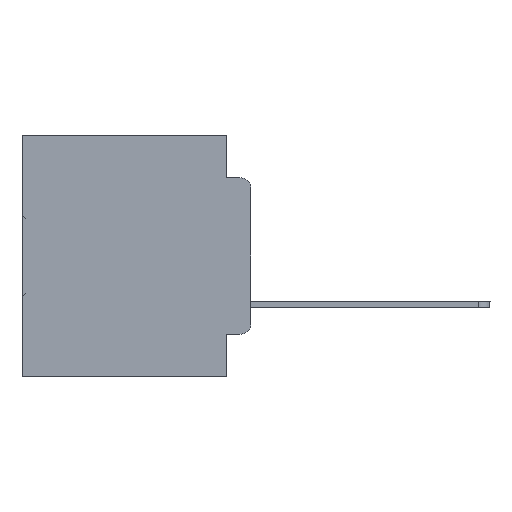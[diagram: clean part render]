
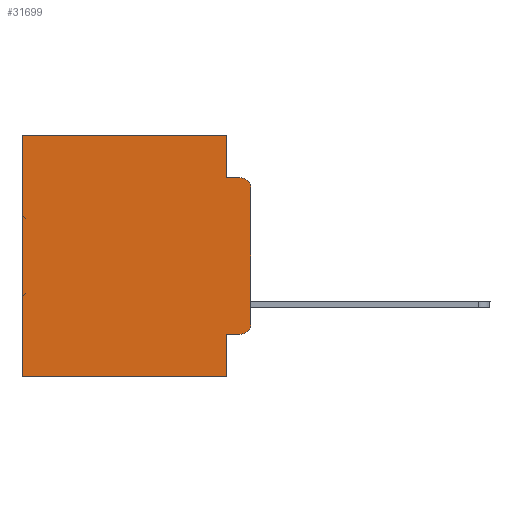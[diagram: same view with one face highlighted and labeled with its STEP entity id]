
A CAD part, left-side view. The second image highlights one B-rep face of the part: STEP entity #31699.
In plain terms, the highlighted planar face has unit normal (-1, 0, 0).
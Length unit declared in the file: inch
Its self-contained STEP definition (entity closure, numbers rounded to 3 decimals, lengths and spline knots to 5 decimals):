
#200 = EDGE_CURVE ( 'NONE', #1109, #8202, #26706, .T. ) ;
#582 = CARTESIAN_POINT ( 'NONE',  ( 0.298, 0.051, 0. ) ) ;
#1109 = VERTEX_POINT ( 'NONE', #20156 ) ;
#1797 = LINE ( 'NONE', #24916, #4919 ) ;
#2735 = CARTESIAN_POINT ( 'NONE',  ( 0.298, 0.02, -0.4115 ) ) ;
#3482 = LINE ( 'NONE', #35218, #13186 ) ;
#3922 = CARTESIAN_POINT ( 'NONE',  ( 0.298, 0.473, 0. ) ) ;
#4274 = ORIENTED_EDGE ( 'NONE', *, *, #35024, .F. ) ;
#4621 = CARTESIAN_POINT ( 'NONE',  ( 0.298, 0., -0.3915 ) ) ;
#4919 = VECTOR ( 'NONE', #36126, 39.37008 ) ;
#4947 = DIRECTION ( 'NONE',  ( 1., 0., 0. ) ) ;
#5190 = DIRECTION ( 'NONE',  ( 0., 0., -1. ) ) ;
#5850 = EDGE_CURVE ( 'NONE', #16998, #13289, #14435, .T. ) ;
#6550 = ORIENTED_EDGE ( 'NONE', *, *, #5850, .F. ) ;
#6618 = CARTESIAN_POINT ( 'NONE',  ( 0.298, 0.051, -0.0885 ) ) ;
#7529 = DIRECTION ( 'NONE',  ( 0., 0., -1. ) ) ;
#7757 = ORIENTED_EDGE ( 'NONE', *, *, #14826, .F. ) ;
#7773 = DIRECTION ( 'NONE',  ( -1., 0., 0. ) ) ;
#8133 = CIRCLE ( 'NONE', #11500, 0.02 ) ;
#8202 = VERTEX_POINT ( 'NONE', #2735 ) ;
#8325 = ORIENTED_EDGE ( 'NONE', *, *, #33126, .T. ) ;
#8741 = DIRECTION ( 'NONE',  ( 0., 1., 0. ) ) ;
#8836 = CARTESIAN_POINT ( 'NONE',  ( 0.298, 0.051, -0.5 ) ) ;
#8849 = LINE ( 'NONE', #16121, #25953 ) ;
#8933 = VERTEX_POINT ( 'NONE', #11521 ) ;
#9349 = DIRECTION ( 'NONE',  ( 0., -1., 0. ) ) ;
#9657 = DIRECTION ( 'NONE',  ( 0., 0., -1. ) ) ;
#10520 = DIRECTION ( 'NONE',  ( 0., 0., -1. ) ) ;
#10917 = VERTEX_POINT ( 'NONE', #8836 ) ;
#11500 = AXIS2_PLACEMENT_3D ( 'NONE', #21645, #7773, #7529 ) ;
#11521 = CARTESIAN_POINT ( 'NONE',  ( 0.298, 0., -0.1085 ) ) ;
#11574 = EDGE_CURVE ( 'NONE', #25132, #14544, #8849, .T. ) ;
#11716 = CARTESIAN_POINT ( 'NONE',  ( 0.298, 0.051, -0.4115 ) ) ;
#12309 = EDGE_LOOP ( 'NONE', ( #17696, #36431, #6550, #28701, #8325, #28999, #4274, #7757, #13156, #26646 ) ) ;
#12980 = CARTESIAN_POINT ( 'NONE',  ( 0.298, 0.02, -0.1085 ) ) ;
#13127 = EDGE_CURVE ( 'NONE', #28359, #16998, #3482, .T. ) ;
#13156 = ORIENTED_EDGE ( 'NONE', *, *, #200, .T. ) ;
#13186 = VECTOR ( 'NONE', #26739, 39.37008 ) ;
#13289 = VERTEX_POINT ( 'NONE', #14630 ) ;
#13422 = DIRECTION ( 'NONE',  ( 0., 0., -1. ) ) ;
#13830 = VECTOR ( 'NONE', #8741, 39.37008 ) ;
#13904 = LINE ( 'NONE', #15154, #35977 ) ;
#14435 = LINE ( 'NONE', #26160, #21106 ) ;
#14544 = VERTEX_POINT ( 'NONE', #21040 ) ;
#14630 = CARTESIAN_POINT ( 'NONE',  ( 0.298, 0.02, -0.0885 ) ) ;
#14826 = EDGE_CURVE ( 'NONE', #1109, #10917, #13904, .T. ) ;
#15154 = CARTESIAN_POINT ( 'NONE',  ( 0.298, 0.051, 0. ) ) ;
#15179 = EDGE_CURVE ( 'NONE', #8933, #13289, #25730, .T. ) ;
#16121 = CARTESIAN_POINT ( 'NONE',  ( 0.298, 0.473, 0. ) ) ;
#16943 = CARTESIAN_POINT ( 'NONE',  ( 0.298, 0., 0. ) ) ;
#16998 = VERTEX_POINT ( 'NONE', #6618 ) ;
#17696 = ORIENTED_EDGE ( 'NONE', *, *, #18624, .F. ) ;
#18624 = EDGE_CURVE ( 'NONE', #8933, #27603, #22601, .T. ) ;
#20156 = CARTESIAN_POINT ( 'NONE',  ( 0.298, 0.051, -0.4115 ) ) ;
#21040 = CARTESIAN_POINT ( 'NONE',  ( 0.298, 0.473, -0.5 ) ) ;
#21106 = VECTOR ( 'NONE', #9349, 39.37008 ) ;
#21639 = CARTESIAN_POINT ( 'NONE',  ( 0.298, 0., 0. ) ) ;
#21645 = CARTESIAN_POINT ( 'NONE',  ( 0.298, 0.02, -0.3915 ) ) ;
#22001 = PLANE ( 'NONE',  #25628 ) ;
#22601 = LINE ( 'NONE', #24983, #23462 ) ;
#22699 = DIRECTION ( 'NONE',  ( 0., -1., 0. ) ) ;
#23462 = VECTOR ( 'NONE', #13422, 39.37008 ) ;
#24916 = CARTESIAN_POINT ( 'NONE',  ( 0.298, 0., -0.5 ) ) ;
#24983 = CARTESIAN_POINT ( 'NONE',  ( 0.298, 0., 0. ) ) ;
#25132 = VERTEX_POINT ( 'NONE', #3922 ) ;
#25628 = AXIS2_PLACEMENT_3D ( 'NONE', #21639, #4947, #5190 ) ;
#25658 = LINE ( 'NONE', #16943, #13830 ) ;
#25730 = CIRCLE ( 'NONE', #34908, 0.02 ) ;
#25953 = VECTOR ( 'NONE', #30619, 39.37008 ) ;
#26160 = CARTESIAN_POINT ( 'NONE',  ( 0.298, 0.051, -0.0885 ) ) ;
#26646 = ORIENTED_EDGE ( 'NONE', *, *, #33498, .T. ) ;
#26706 = LINE ( 'NONE', #11716, #29786 ) ;
#26739 = DIRECTION ( 'NONE',  ( 0., 0., -1. ) ) ;
#27603 = VERTEX_POINT ( 'NONE', #4621 ) ;
#28359 = VERTEX_POINT ( 'NONE', #582 ) ;
#28701 = ORIENTED_EDGE ( 'NONE', *, *, #13127, .F. ) ;
#28999 = ORIENTED_EDGE ( 'NONE', *, *, #11574, .T. ) ;
#29786 = VECTOR ( 'NONE', #22699, 39.37008 ) ;
#30619 = DIRECTION ( 'NONE',  ( 0., 0., -1. ) ) ;
#31699 = ADVANCED_FACE ( 'NONE', ( #35961 ), #22001, .F. ) ;
#33126 = EDGE_CURVE ( 'NONE', #28359, #25132, #25658, .T. ) ;
#33498 = EDGE_CURVE ( 'NONE', #8202, #27603, #8133, .T. ) ;
#34908 = AXIS2_PLACEMENT_3D ( 'NONE', #12980, #35753, #10520 ) ;
#35024 = EDGE_CURVE ( 'NONE', #10917, #14544, #1797, .T. ) ;
#35218 = CARTESIAN_POINT ( 'NONE',  ( 0.298, 0.051, 0. ) ) ;
#35753 = DIRECTION ( 'NONE',  ( -1., 0., 0. ) ) ;
#35961 = FACE_OUTER_BOUND ( 'NONE', #12309, .T. ) ;
#35977 = VECTOR ( 'NONE', #9657, 39.37008 ) ;
#36126 = DIRECTION ( 'NONE',  ( 0., 1., 0. ) ) ;
#36431 = ORIENTED_EDGE ( 'NONE', *, *, #15179, .T. ) ;
